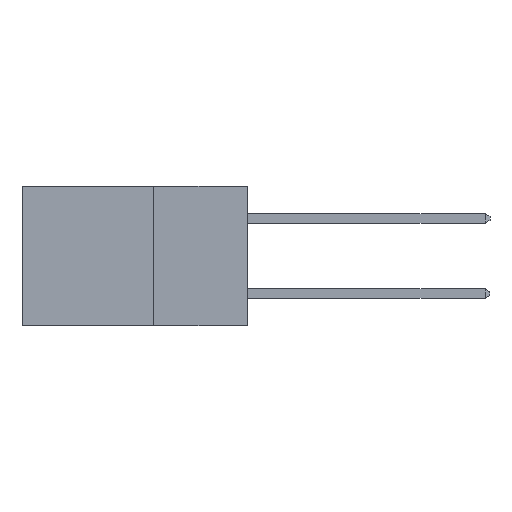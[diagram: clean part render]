
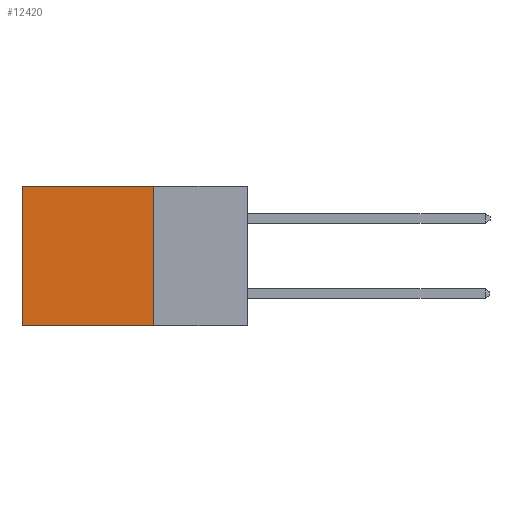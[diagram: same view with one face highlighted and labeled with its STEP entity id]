
A CAD part, left-side view. The second image highlights one B-rep face of the part: STEP entity #12420.
In plain terms, the highlighted planar face has unit normal (-1, 0, 0).
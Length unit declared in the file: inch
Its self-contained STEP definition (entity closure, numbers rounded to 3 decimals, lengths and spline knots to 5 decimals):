
#135 = DIRECTION ( 'NONE',  ( 0., 0., -1. ) ) ;
#261 = VECTOR ( 'NONE', #8819, 39.37008 ) ;
#500 = EDGE_CURVE ( 'NONE', #17075, #11876, #24909, .T. ) ;
#945 = LINE ( 'NONE', #10957, #261 ) ;
#1228 = CARTESIAN_POINT ( 'NONE',  ( 0.298, 0.25, -0.37 ) ) ;
#2517 = DIRECTION ( 'NONE',  ( 0., 0., -1. ) ) ;
#2525 = VERTEX_POINT ( 'NONE', #12153 ) ;
#2734 = ORIENTED_EDGE ( 'NONE', *, *, #500, .F. ) ;
#2825 = EDGE_CURVE ( 'NONE', #19743, #17075, #11682, .T. ) ;
#4218 = EDGE_CURVE ( 'NONE', #2525, #11876, #9990, .T. ) ;
#4377 = EDGE_CURVE ( 'NONE', #19743, #2525, #945, .T. ) ;
#5393 = DIRECTION ( 'NONE',  ( 0., 1., 0. ) ) ;
#8819 = DIRECTION ( 'NONE',  ( 0., 1., 0. ) ) ;
#9990 = LINE ( 'NONE', #21051, #21165 ) ;
#10371 = VECTOR ( 'NONE', #2517, 39.37008 ) ;
#10814 = CARTESIAN_POINT ( 'NONE',  ( 0.298, 0.25, 0. ) ) ;
#10957 = CARTESIAN_POINT ( 'NONE',  ( 0.298, 0.25, 0. ) ) ;
#11682 = LINE ( 'NONE', #17373, #10371 ) ;
#11876 = VERTEX_POINT ( 'NONE', #23453 ) ;
#12153 = CARTESIAN_POINT ( 'NONE',  ( 0.298, 0.6, 0. ) ) ;
#12420 = ADVANCED_FACE ( 'NONE', ( #21127 ), #23352, .F. ) ;
#12950 = DIRECTION ( 'NONE',  ( 1., 0., 0. ) ) ;
#17075 = VERTEX_POINT ( 'NONE', #1228 ) ;
#17373 = CARTESIAN_POINT ( 'NONE',  ( 0.298, 0.25, 0. ) ) ;
#18650 = ORIENTED_EDGE ( 'NONE', *, *, #4218, .T. ) ;
#19743 = VERTEX_POINT ( 'NONE', #24676 ) ;
#20728 = EDGE_LOOP ( 'NONE', ( #18650, #2734, #21041, #27070 ) ) ;
#21041 = ORIENTED_EDGE ( 'NONE', *, *, #2825, .F. ) ;
#21051 = CARTESIAN_POINT ( 'NONE',  ( 0.298, 0.6, 0. ) ) ;
#21127 = FACE_OUTER_BOUND ( 'NONE', #20728, .T. ) ;
#21165 = VECTOR ( 'NONE', #23135, 39.37008 ) ;
#23135 = DIRECTION ( 'NONE',  ( 0., 0., -1. ) ) ;
#23352 = PLANE ( 'NONE',  #23754 ) ;
#23453 = CARTESIAN_POINT ( 'NONE',  ( 0.298, 0.6, -0.37 ) ) ;
#23608 = VECTOR ( 'NONE', #5393, 39.37008 ) ;
#23754 = AXIS2_PLACEMENT_3D ( 'NONE', #10814, #12950, #135 ) ;
#24086 = CARTESIAN_POINT ( 'NONE',  ( 0.298, 0.25, -0.37 ) ) ;
#24676 = CARTESIAN_POINT ( 'NONE',  ( 0.298, 0.25, 0. ) ) ;
#24909 = LINE ( 'NONE', #24086, #23608 ) ;
#27070 = ORIENTED_EDGE ( 'NONE', *, *, #4377, .T. ) ;
